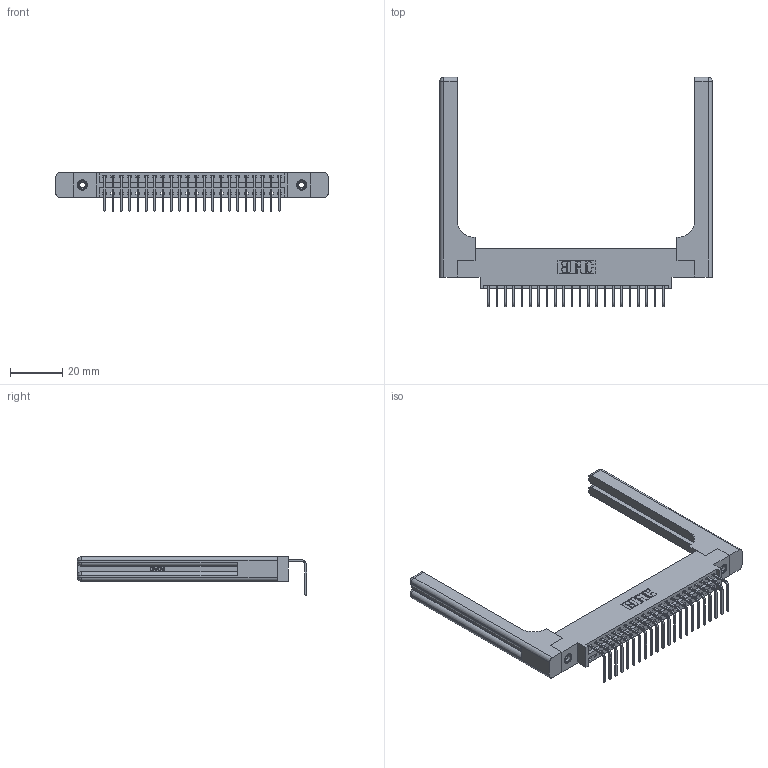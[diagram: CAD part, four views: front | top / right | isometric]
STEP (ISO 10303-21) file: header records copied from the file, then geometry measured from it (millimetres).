
FILE_DESCRIPTION (( 'STEP AP203' ), '1' );
FILE_NAME ('396-022-558-658.STEP', '2019-11-01T06:20:02', ( '' ), ( '' ), 'SwSTEP 2.0', 'SolidWorks 2016', '' );
FILE_SCHEMA (( 'CONFIG_CONTROL_DESIGN' ));
Length unit declared in the file: inch
Products named in the file (5): 346 Part_0.170 Offset - 0.156 Dia-TH; 345-292-001_558 Tail - 2; 345-250-001_345-250-001-102; 346-220-058_345-220-058; 396-022-558-658
Assembly tree (27 placements, depth 2):
  396-022-558-658
    346 Part_0.170 Offset - 0.156 Dia-TH
    345-292-001_558 Tail - 2  x22
    345-250-001_345-250-001-102  x2
    346-220-058_345-220-058  x2
Bounding box: 103.91 x 87.44 x 14.73 mm (x, y, z)
Volume: 17245.9 mm3; surface area: 17709.5 mm2
Topology: 27 solids, 27 shells, 1702 faces, 5011 edges, 3290 vertices
Faces by surface type: plane 1152, cylinder 490, bspline 36, cone 12, sphere 8, torus 4
Entity records: 21744 total; most frequent: CARTESIAN_POINT 4715, ORIENTED_EDGE 3468, DIRECTION 3114, EDGE_CURVE 1734, LINE 1422, VECTOR 1422, VERTEX_POINT 1146, AXIS2_PLACEMENT_3D 846
